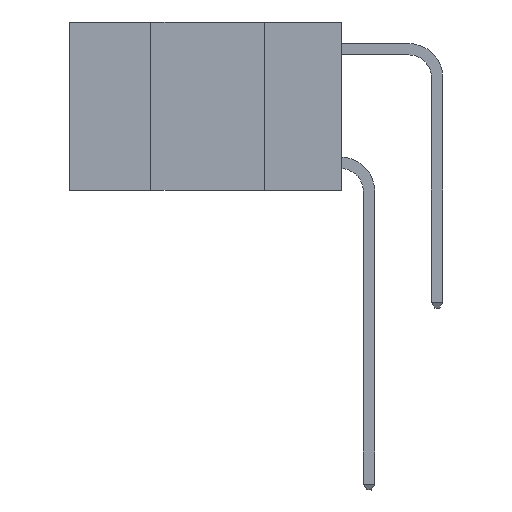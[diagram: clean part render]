
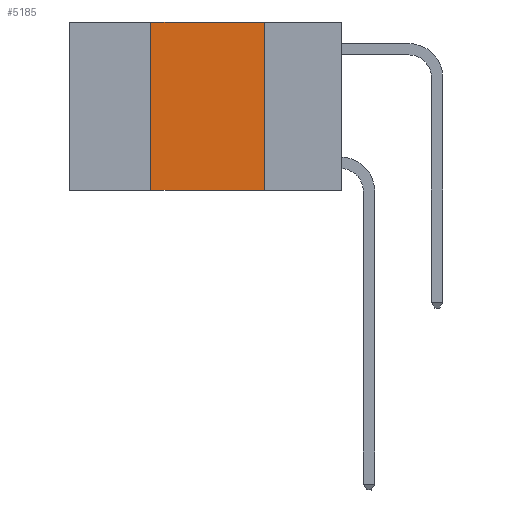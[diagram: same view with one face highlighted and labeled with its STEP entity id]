
A CAD part, left-side view. The second image highlights one B-rep face of the part: STEP entity #5185.
In plain terms, the highlighted planar face has unit normal (-1, 0, 0).
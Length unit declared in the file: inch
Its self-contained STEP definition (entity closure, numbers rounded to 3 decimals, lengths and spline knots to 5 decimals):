
#774 = ORIENTED_EDGE ( 'NONE', *, *, #7092, .F. ) ;
#1177 = ORIENTED_EDGE ( 'NONE', *, *, #15380, .F. ) ;
#1330 = VERTEX_POINT ( 'NONE', #14922 ) ;
#1536 = CARTESIAN_POINT ( 'NONE',  ( 0., 0.42, 0. ) ) ;
#1721 = VECTOR ( 'NONE', #7263, 39.37008 ) ;
#2525 = CARTESIAN_POINT ( 'NONE',  ( 0., 0.6, 0. ) ) ;
#3279 = LINE ( 'NONE', #12674, #15683 ) ;
#3473 = VERTEX_POINT ( 'NONE', #1536 ) ;
#4770 = ORIENTED_EDGE ( 'NONE', *, *, #13320, .T. ) ;
#5185 = ADVANCED_FACE ( 'NONE', ( #12102 ), #7557, .F. ) ;
#5214 = DIRECTION ( 'NONE',  ( 0., 0., -1. ) ) ;
#5889 = EDGE_CURVE ( 'NONE', #3473, #13735, #8999, .T. ) ;
#7092 = EDGE_CURVE ( 'NONE', #13735, #1330, #11515, .T. ) ;
#7263 = DIRECTION ( 'NONE',  ( 0., 0., 1. ) ) ;
#7395 = CARTESIAN_POINT ( 'NONE',  ( 0., 0.17, 0. ) ) ;
#7557 = PLANE ( 'NONE',  #15594 ) ;
#7638 = ORIENTED_EDGE ( 'NONE', *, *, #5889, .F. ) ;
#8333 = DIRECTION ( 'NONE',  ( 0., 0., -1. ) ) ;
#8403 = VERTEX_POINT ( 'NONE', #12552 ) ;
#8781 = CARTESIAN_POINT ( 'NONE',  ( 0., 0.6, 0. ) ) ;
#8999 = LINE ( 'NONE', #2525, #11730 ) ;
#11515 = LINE ( 'NONE', #13056, #14655 ) ;
#11730 = VECTOR ( 'NONE', #13479, 39.37008 ) ;
#12102 = FACE_OUTER_BOUND ( 'NONE', #15857, .T. ) ;
#12305 = DIRECTION ( 'NONE',  ( 1., 0., 0. ) ) ;
#12552 = CARTESIAN_POINT ( 'NONE',  ( 0., 0.42, -0.37 ) ) ;
#12674 = CARTESIAN_POINT ( 'NONE',  ( 0., 0.6, -0.37 ) ) ;
#13056 = CARTESIAN_POINT ( 'NONE',  ( 0., 0.17, 0. ) ) ;
#13119 = CARTESIAN_POINT ( 'NONE',  ( 0., 0.42, 0. ) ) ;
#13320 = EDGE_CURVE ( 'NONE', #8403, #1330, #3279, .T. ) ;
#13479 = DIRECTION ( 'NONE',  ( 0., -1., 0. ) ) ;
#13735 = VERTEX_POINT ( 'NONE', #7395 ) ;
#13860 = DIRECTION ( 'NONE',  ( 0., -1., 0. ) ) ;
#14655 = VECTOR ( 'NONE', #8333, 39.37008 ) ;
#14922 = CARTESIAN_POINT ( 'NONE',  ( 0., 0.17, -0.37 ) ) ;
#15087 = LINE ( 'NONE', #13119, #1721 ) ;
#15380 = EDGE_CURVE ( 'NONE', #8403, #3473, #15087, .T. ) ;
#15594 = AXIS2_PLACEMENT_3D ( 'NONE', #8781, #12305, #5214 ) ;
#15683 = VECTOR ( 'NONE', #13860, 39.37008 ) ;
#15857 = EDGE_LOOP ( 'NONE', ( #774, #7638, #1177, #4770 ) ) ;
